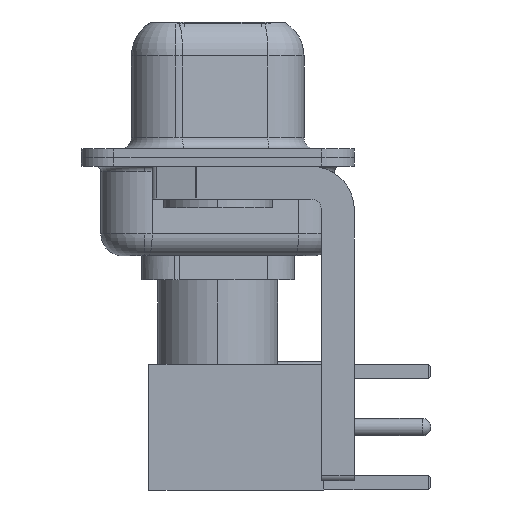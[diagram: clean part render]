
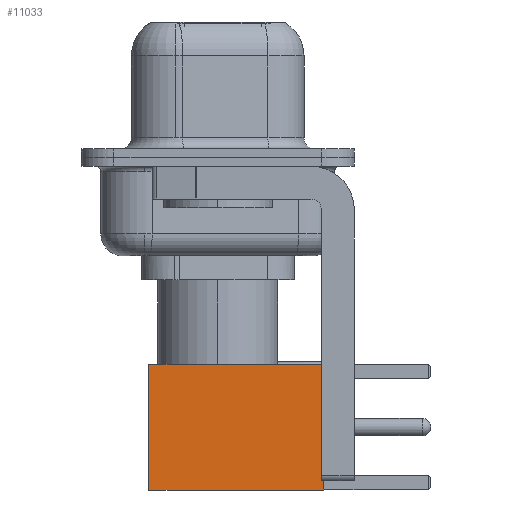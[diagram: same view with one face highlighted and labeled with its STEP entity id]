
A CAD part, left-side view. The second image highlights one B-rep face of the part: STEP entity #11033.
In plain terms, the highlighted face is planar.
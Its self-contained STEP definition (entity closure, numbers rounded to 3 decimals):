
#20 = EDGE_CURVE ( 'NONE', #4596, #7293, #11648, .T. ) ;
#2035 = VECTOR ( 'NONE', #18680, 1000. ) ;
#2108 = VERTEX_POINT ( 'NONE', #10769 ) ;
#2935 = DIRECTION ( 'NONE',  ( 0., 0., -1. ) ) ;
#4596 = VERTEX_POINT ( 'NONE', #19872 ) ;
#4749 = LINE ( 'NONE', #16408, #2035 ) ;
#5065 = VECTOR ( 'NONE', #19986, 1000. ) ;
#6048 = EDGE_CURVE ( 'NONE', #4596, #18392, #19618, .T. ) ;
#7293 = VERTEX_POINT ( 'NONE', #11565 ) ;
#7965 = CARTESIAN_POINT ( 'NONE',  ( 2.875, 2.875, 0. ) ) ;
#8029 = DIRECTION ( 'NONE',  ( 0., 0., 1. ) ) ;
#8963 = VECTOR ( 'NONE', #19360, 1000. ) ;
#9017 = LINE ( 'NONE', #20539, #21251 ) ;
#10769 = CARTESIAN_POINT ( 'NONE',  ( -2.875, 2.875, 0. ) ) ;
#11033 = ADVANCED_FACE ( 'NONE', ( #13872 ), #15631, .T. ) ;
#11565 = CARTESIAN_POINT ( 'NONE',  ( -2.875, 2.875, 8. ) ) ;
#11648 = LINE ( 'NONE', #23140, #8963 ) ;
#12665 = ORIENTED_EDGE ( 'NONE', *, *, #22347, .T. ) ;
#13160 = ORIENTED_EDGE ( 'NONE', *, *, #17395, .F. ) ;
#13872 = FACE_OUTER_BOUND ( 'NONE', #14829, .T. ) ;
#13994 = DIRECTION ( 'NONE',  ( 0., 1., 0. ) ) ;
#14829 = EDGE_LOOP ( 'NONE', ( #19520, #12665, #13160, #18839 ) ) ;
#15631 = PLANE ( 'NONE',  #23823 ) ;
#16408 = CARTESIAN_POINT ( 'NONE',  ( 0., 2.875, 0. ) ) ;
#17395 = EDGE_CURVE ( 'NONE', #7293, #2108, #9017, .T. ) ;
#18392 = VERTEX_POINT ( 'NONE', #22243 ) ;
#18680 = DIRECTION ( 'NONE',  ( -1., 0., 0. ) ) ;
#18839 = ORIENTED_EDGE ( 'NONE', *, *, #20, .F. ) ;
#19360 = DIRECTION ( 'NONE',  ( -1., 0., 0. ) ) ;
#19520 = ORIENTED_EDGE ( 'NONE', *, *, #6048, .T. ) ;
#19618 = LINE ( 'NONE', #7965, #5065 ) ;
#19872 = CARTESIAN_POINT ( 'NONE',  ( 2.875, 2.875, 8. ) ) ;
#19986 = DIRECTION ( 'NONE',  ( 0., 0., -1. ) ) ;
#20539 = CARTESIAN_POINT ( 'NONE',  ( -2.875, 2.875, 0. ) ) ;
#21251 = VECTOR ( 'NONE', #2935, 1000. ) ;
#21683 = CARTESIAN_POINT ( 'NONE',  ( 2.875, 2.875, 0. ) ) ;
#22243 = CARTESIAN_POINT ( 'NONE',  ( 2.875, 2.875, 0. ) ) ;
#22347 = EDGE_CURVE ( 'NONE', #18392, #2108, #4749, .T. ) ;
#23140 = CARTESIAN_POINT ( 'NONE',  ( 0., 2.875, 8. ) ) ;
#23823 = AXIS2_PLACEMENT_3D ( 'NONE', #21683, #13994, #8029 ) ;
